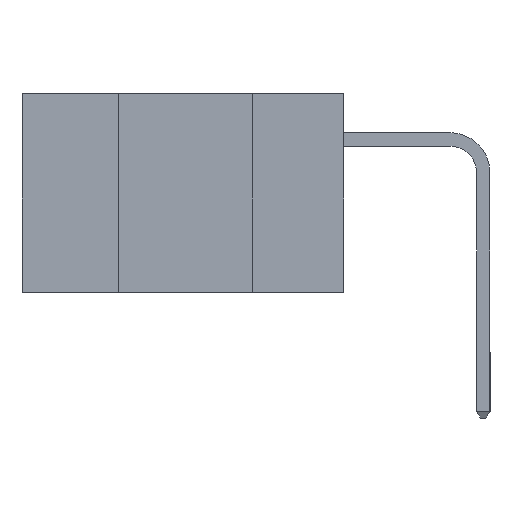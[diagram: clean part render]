
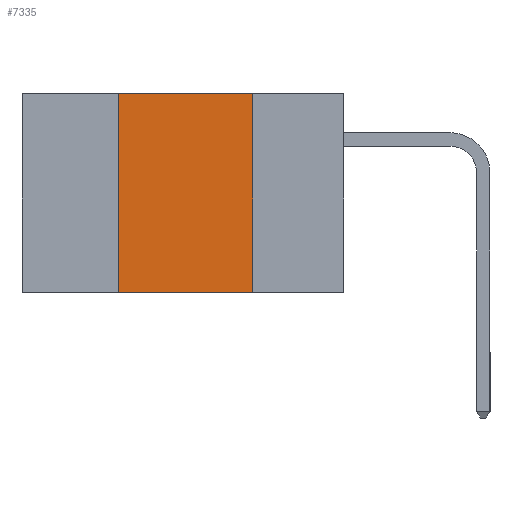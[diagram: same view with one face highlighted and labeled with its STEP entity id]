
A CAD part, left-side view. The second image highlights one B-rep face of the part: STEP entity #7335.
In plain terms, the highlighted planar face has unit normal (-1, 0, 0).
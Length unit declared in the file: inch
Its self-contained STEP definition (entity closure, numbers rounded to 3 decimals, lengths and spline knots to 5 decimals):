
#707 = VERTEX_POINT ( 'NONE', #13091 ) ;
#945 = DIRECTION ( 'NONE',  ( 0., 0., 1. ) ) ;
#1221 = EDGE_CURVE ( 'NONE', #707, #9868, #8039, .T. ) ;
#1522 = CARTESIAN_POINT ( 'NONE',  ( 0., 0.42, -0.37 ) ) ;
#2977 = FACE_OUTER_BOUND ( 'NONE', #15659, .T. ) ;
#3123 = ORIENTED_EDGE ( 'NONE', *, *, #15508, .T. ) ;
#3379 = CARTESIAN_POINT ( 'NONE',  ( 0., 0.17, 0. ) ) ;
#3924 = VECTOR ( 'NONE', #8741, 39.37008 ) ;
#3974 = CARTESIAN_POINT ( 'NONE',  ( 0., 0.6, 0. ) ) ;
#4160 = AXIS2_PLACEMENT_3D ( 'NONE', #3974, #13834, #11062 ) ;
#4263 = CARTESIAN_POINT ( 'NONE',  ( 0., 0.17, -0.37 ) ) ;
#5272 = VERTEX_POINT ( 'NONE', #4263 ) ;
#6933 = PLANE ( 'NONE',  #4160 ) ;
#6943 = LINE ( 'NONE', #12684, #3924 ) ;
#7335 = ADVANCED_FACE ( 'NONE', ( #2977 ), #6933, .F. ) ;
#8039 = LINE ( 'NONE', #13754, #17267 ) ;
#8741 = DIRECTION ( 'NONE',  ( 0., -1., 0. ) ) ;
#9038 = LINE ( 'NONE', #14472, #10819 ) ;
#9640 = DIRECTION ( 'NONE',  ( 0., -1., 0. ) ) ;
#9846 = ORIENTED_EDGE ( 'NONE', *, *, #1221, .F. ) ;
#9868 = VERTEX_POINT ( 'NONE', #3379 ) ;
#10008 = ORIENTED_EDGE ( 'NONE', *, *, #15326, .F. ) ;
#10454 = EDGE_CURVE ( 'NONE', #9868, #5272, #12237, .T. ) ;
#10819 = VECTOR ( 'NONE', #945, 39.37008 ) ;
#10891 = CARTESIAN_POINT ( 'NONE',  ( 0., 0.17, -0.37 ) ) ;
#11062 = DIRECTION ( 'NONE',  ( 0., 0., -1. ) ) ;
#12237 = LINE ( 'NONE', #10891, #17287 ) ;
#12684 = CARTESIAN_POINT ( 'NONE',  ( 0., 0.6, -0.37 ) ) ;
#13091 = CARTESIAN_POINT ( 'NONE',  ( 0., 0.42, 0. ) ) ;
#13754 = CARTESIAN_POINT ( 'NONE',  ( 0., 0.6, 0. ) ) ;
#13834 = DIRECTION ( 'NONE',  ( 1., 0., 0. ) ) ;
#14472 = CARTESIAN_POINT ( 'NONE',  ( 0., 0.42, -0.37 ) ) ;
#14690 = VERTEX_POINT ( 'NONE', #1522 ) ;
#14991 = ORIENTED_EDGE ( 'NONE', *, *, #10454, .F. ) ;
#15224 = DIRECTION ( 'NONE',  ( 0., 0., -1. ) ) ;
#15326 = EDGE_CURVE ( 'NONE', #14690, #707, #9038, .T. ) ;
#15508 = EDGE_CURVE ( 'NONE', #14690, #5272, #6943, .T. ) ;
#15659 = EDGE_LOOP ( 'NONE', ( #14991, #9846, #10008, #3123 ) ) ;
#17267 = VECTOR ( 'NONE', #9640, 39.37008 ) ;
#17287 = VECTOR ( 'NONE', #15224, 39.37008 ) ;
